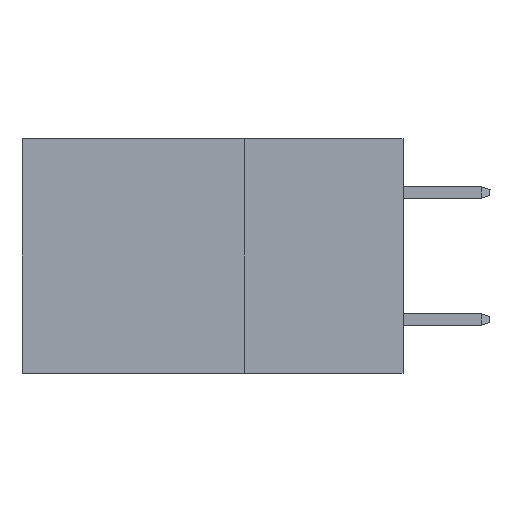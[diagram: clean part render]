
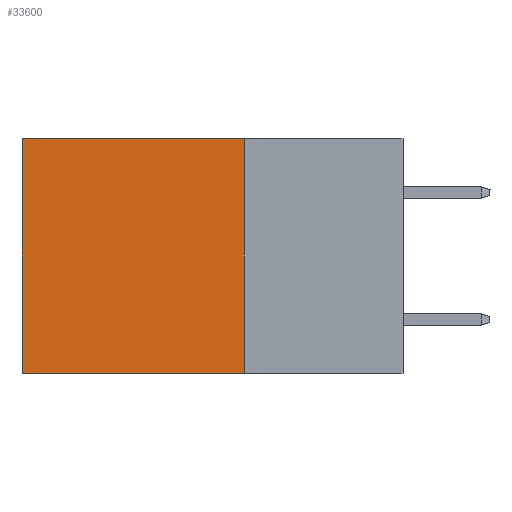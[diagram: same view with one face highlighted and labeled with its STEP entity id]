
A CAD part, left-side view. The second image highlights one B-rep face of the part: STEP entity #33600.
In plain terms, the highlighted planar face has unit normal (-1, 0, 0).
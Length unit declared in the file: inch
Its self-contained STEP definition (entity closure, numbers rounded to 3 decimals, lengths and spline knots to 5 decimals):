
#2745 = DIRECTION ( 'NONE',  ( 0., 0., -1. ) ) ;
#3213 = VERTEX_POINT ( 'NONE', #33718 ) ;
#3494 = VECTOR ( 'NONE', #25374, 39.37008 ) ;
#5942 = ORIENTED_EDGE ( 'NONE', *, *, #12978, .T. ) ;
#7061 = LINE ( 'NONE', #12768, #3494 ) ;
#7110 = VECTOR ( 'NONE', #38364, 39.37008 ) ;
#7626 = LINE ( 'NONE', #37762, #7110 ) ;
#8361 = ORIENTED_EDGE ( 'NONE', *, *, #34826, .F. ) ;
#11524 = PLANE ( 'NONE',  #26679 ) ;
#12344 = CARTESIAN_POINT ( 'NONE',  ( 0.2875, 0.6, 0. ) ) ;
#12768 = CARTESIAN_POINT ( 'NONE',  ( 0.2875, 0.25, -0.37 ) ) ;
#12978 = EDGE_CURVE ( 'NONE', #18243, #29313, #15796, .T. ) ;
#15796 = LINE ( 'NONE', #12344, #33246 ) ;
#16822 = CARTESIAN_POINT ( 'NONE',  ( 0.2875, 0.6, 0. ) ) ;
#17999 = EDGE_CURVE ( 'NONE', #3213, #29313, #7061, .T. ) ;
#18243 = VERTEX_POINT ( 'NONE', #16822 ) ;
#20095 = ORIENTED_EDGE ( 'NONE', *, *, #30556, .T. ) ;
#22670 = CARTESIAN_POINT ( 'NONE',  ( 0.2875, 0.25, 0. ) ) ;
#24326 = CARTESIAN_POINT ( 'NONE',  ( 0.2875, 0.25, 0. ) ) ;
#25052 = ORIENTED_EDGE ( 'NONE', *, *, #17999, .F. ) ;
#25374 = DIRECTION ( 'NONE',  ( 0., 1., 0. ) ) ;
#26003 = EDGE_LOOP ( 'NONE', ( #5942, #25052, #8361, #20095 ) ) ;
#26382 = DIRECTION ( 'NONE',  ( 0., 0., -1. ) ) ;
#26679 = AXIS2_PLACEMENT_3D ( 'NONE', #24326, #30442, #2745 ) ;
#28939 = CARTESIAN_POINT ( 'NONE',  ( 0.2875, 0.6, -0.37 ) ) ;
#29313 = VERTEX_POINT ( 'NONE', #28939 ) ;
#30442 = DIRECTION ( 'NONE',  ( 1., 0., 0. ) ) ;
#30556 = EDGE_CURVE ( 'NONE', #35208, #18243, #7626, .T. ) ;
#32687 = LINE ( 'NONE', #38600, #38449 ) ;
#33173 = DIRECTION ( 'NONE',  ( 0., 0., -1. ) ) ;
#33246 = VECTOR ( 'NONE', #33173, 39.37008 ) ;
#33600 = ADVANCED_FACE ( 'NONE', ( #39606 ), #11524, .F. ) ;
#33718 = CARTESIAN_POINT ( 'NONE',  ( 0.2875, 0.25, -0.37 ) ) ;
#34826 = EDGE_CURVE ( 'NONE', #35208, #3213, #32687, .T. ) ;
#35208 = VERTEX_POINT ( 'NONE', #22670 ) ;
#37762 = CARTESIAN_POINT ( 'NONE',  ( 0.2875, 0.25, 0. ) ) ;
#38364 = DIRECTION ( 'NONE',  ( 0., 1., 0. ) ) ;
#38449 = VECTOR ( 'NONE', #26382, 39.37008 ) ;
#38600 = CARTESIAN_POINT ( 'NONE',  ( 0.2875, 0.25, 0. ) ) ;
#39606 = FACE_OUTER_BOUND ( 'NONE', #26003, .T. ) ;
